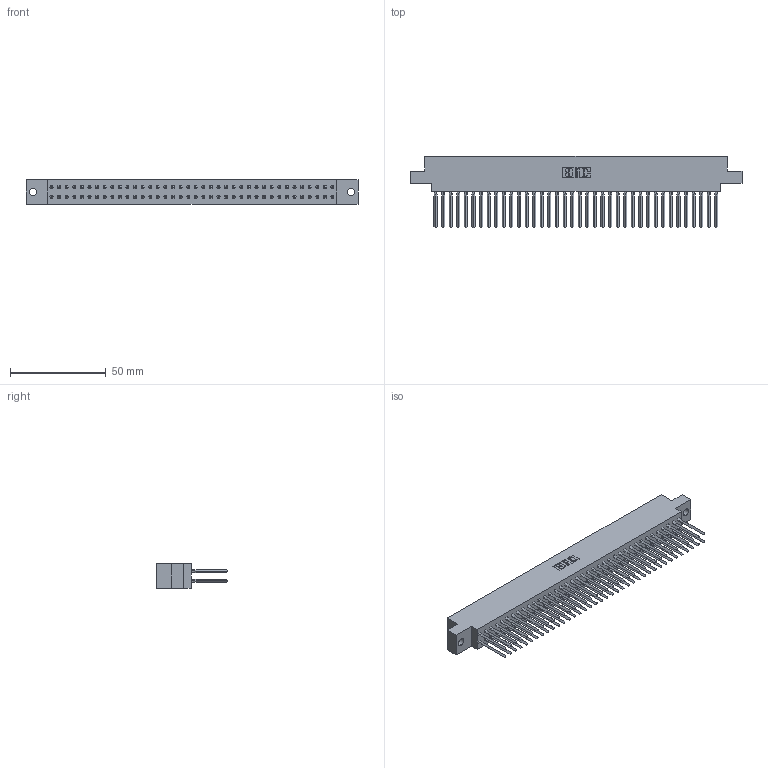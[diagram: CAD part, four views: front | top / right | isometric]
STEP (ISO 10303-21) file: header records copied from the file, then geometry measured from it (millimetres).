
FILE_DESCRIPTION (( 'STEP AP203' ), '1' );
FILE_NAME ('317-076-540-804.STEP', '2020-02-28T08:15:41', ( '' ), ( '' ), 'SwSTEP 2.0', 'SolidWorks 2016', '' );
FILE_SCHEMA (( 'CONFIG_CONTROL_DESIGN' ));
Length unit declared in the file: inch
Products named in the file (3): 317 Part_.156 Dia - TH; 317-076-540-804; 317-290-001_540
Assembly tree (77 placements, depth 2):
  317-076-540-804
    317 Part_.156 Dia - TH
    317-290-001_540  x76
Bounding box: 173.28 x 37.34 x 12.7 mm (x, y, z)
Volume: 28858.5 mm3; surface area: 42699.4 mm2
Topology: 77 solids, 77 shells, 6866 faces, 19047 edges, 12266 vertices
Faces by surface type: plane 5606, cylinder 956, bspline 304
Entity records: 55490 total; most frequent: CARTESIAN_POINT 10095, ORIENTED_EDGE 9594, DIRECTION 8003, EDGE_CURVE 4797, LINE 4541, VECTOR 4541, VERTEX_POINT 3191, AXIS2_PLACEMENT_3D 1731
